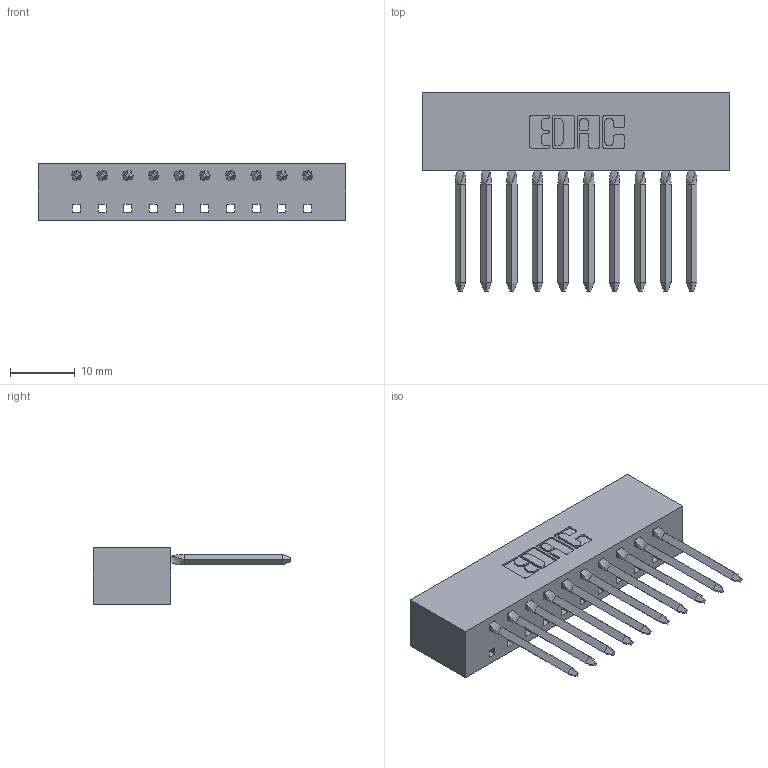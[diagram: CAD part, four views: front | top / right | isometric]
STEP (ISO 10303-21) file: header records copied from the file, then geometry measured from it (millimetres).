
FILE_DESCRIPTION (( 'STEP AP203' ), '1' );
FILE_NAME ('338-010-541-101.STEP', '2020-03-24T16:53:43', ( '' ), ( '' ), 'SwSTEP 2.0', 'SolidWorks 2016', '' );
FILE_SCHEMA (( 'CONFIG_CONTROL_DESIGN' ));
Length unit declared in the file: inch
Products named in the file (3): 338-290-001_541; 338-210-001_338-210-010-001; 338-010-541-101
Assembly tree (11 placements, depth 2):
  338-010-541-101
    338-210-001_338-210-010-001
    338-290-001_541  x10
Bounding box: 47.5 x 30.56 x 8.71 mm (x, y, z)
Volume: 3568 mm3; surface area: 5593.4 mm2
Topology: 11 solids, 11 shells, 1016 faces, 2797 edges, 1790 vertices
Faces by surface type: plane 696, cylinder 280, bspline 40
Entity records: 22326 total; most frequent: CARTESIAN_POINT 4566, ORIENTED_EDGE 3740, DIRECTION 3469, EDGE_CURVE 1870, VECTOR 1347, LINE 1347, VERTEX_POINT 1214, AXIS2_PLACEMENT_3D 1061
